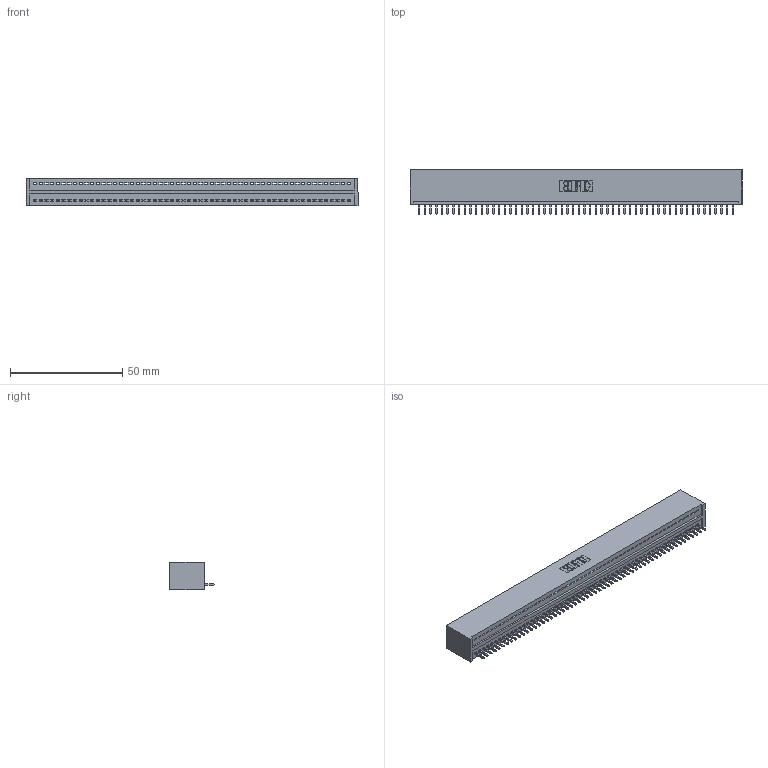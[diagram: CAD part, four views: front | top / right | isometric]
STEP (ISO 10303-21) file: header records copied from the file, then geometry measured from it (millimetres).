
FILE_DESCRIPTION (( 'STEP AP203' ), '1' );
FILE_NAME ('325-056-520-101.STEP', '2020-02-25T01:24:09', ( '' ), ( '' ), 'SwSTEP 2.0', 'SolidWorks 2016', '' );
FILE_SCHEMA (( 'CONFIG_CONTROL_DESIGN' ));
Length unit declared in the file: inch
Products named in the file (3): 325 Part_Lugless; 325-056-520-101; 325-292-001_325-293-120
Assembly tree (57 placements, depth 2):
  325-056-520-101
    325 Part_Lugless
    325-292-001_325-293-120  x56
Bounding box: 147.88 x 19.68 x 12.45 mm (x, y, z)
Volume: 19310.3 mm3; surface area: 21235.5 mm2
Topology: 57 solids, 57 shells, 3354 faces, 10143 edges, 6686 vertices
Faces by surface type: plane 2418, cylinder 936
Entity records: 32165 total; most frequent: CARTESIAN_POINT 5554, ORIENTED_EDGE 5546, DIRECTION 4649, EDGE_CURVE 2773, VECTOR 2653, LINE 2653, VERTEX_POINT 1846, AXIS2_PLACEMENT_3D 998
